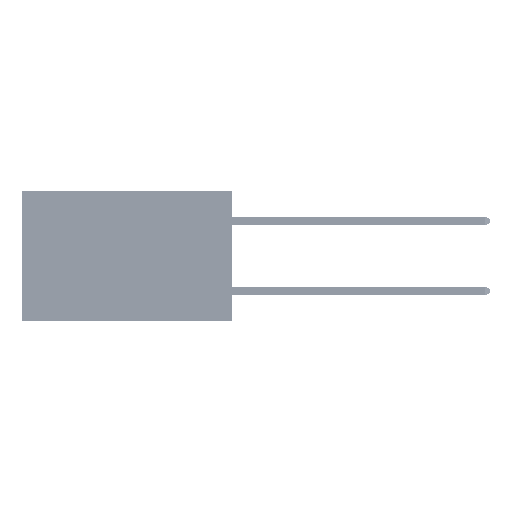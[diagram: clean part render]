
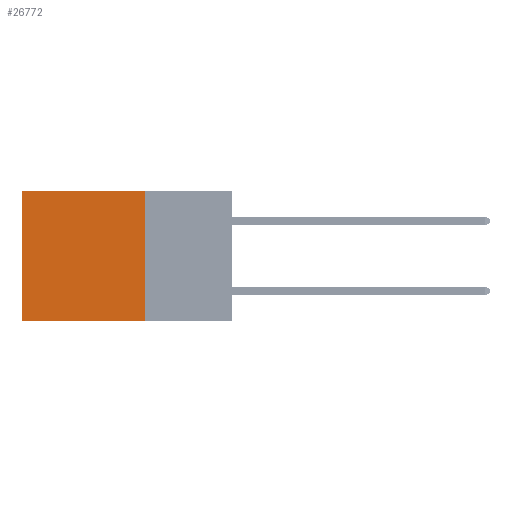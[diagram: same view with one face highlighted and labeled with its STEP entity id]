
A CAD part, left-side view. The second image highlights one B-rep face of the part: STEP entity #26772.
In plain terms, the highlighted planar face has unit normal (-1, 0, 0).
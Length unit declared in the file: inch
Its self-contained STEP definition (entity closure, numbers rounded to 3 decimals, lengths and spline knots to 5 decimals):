
#1401 = LINE ( 'NONE', #15928, #24816 ) ;
#1946 = AXIS2_PLACEMENT_3D ( 'NONE', #35711, #35251, #28089 ) ;
#4769 = ORIENTED_EDGE ( 'NONE', *, *, #20367, .F. ) ;
#4909 = CARTESIAN_POINT ( 'NONE',  ( 0.2875, 0.25, -0.37 ) ) ;
#7418 = EDGE_CURVE ( 'NONE', #21669, #17440, #38438, .T. ) ;
#8050 = EDGE_LOOP ( 'NONE', ( #38858, #29986, #4769, #27106 ) ) ;
#8296 = VERTEX_POINT ( 'NONE', #4909 ) ;
#8404 = DIRECTION ( 'NONE',  ( 0., 1., 0. ) ) ;
#8868 = CARTESIAN_POINT ( 'NONE',  ( 0.2875, 0.25, 0. ) ) ;
#14038 = VERTEX_POINT ( 'NONE', #43383 ) ;
#14043 = CARTESIAN_POINT ( 'NONE',  ( 0.2875, 0.6, 0. ) ) ;
#15928 = CARTESIAN_POINT ( 'NONE',  ( 0.2875, 0.25, -0.37 ) ) ;
#17440 = VERTEX_POINT ( 'NONE', #37973 ) ;
#18026 = EDGE_CURVE ( 'NONE', #17440, #14038, #46707, .T. ) ;
#18798 = VECTOR ( 'NONE', #8404, 39.37008 ) ;
#20367 = EDGE_CURVE ( 'NONE', #21669, #8296, #30829, .T. ) ;
#21669 = VERTEX_POINT ( 'NONE', #40233 ) ;
#23200 = CARTESIAN_POINT ( 'NONE',  ( 0.2875, 0.25, 0. ) ) ;
#24816 = VECTOR ( 'NONE', #45004, 39.37008 ) ;
#26772 = ADVANCED_FACE ( 'NONE', ( #31207 ), #46192, .F. ) ;
#27106 = ORIENTED_EDGE ( 'NONE', *, *, #7418, .T. ) ;
#28089 = DIRECTION ( 'NONE',  ( 0., 0., -1. ) ) ;
#28594 = DIRECTION ( 'NONE',  ( 0., 0., -1. ) ) ;
#29986 = ORIENTED_EDGE ( 'NONE', *, *, #46075, .F. ) ;
#30829 = LINE ( 'NONE', #23200, #34383 ) ;
#31207 = FACE_OUTER_BOUND ( 'NONE', #8050, .T. ) ;
#32213 = VECTOR ( 'NONE', #28594, 39.37008 ) ;
#34383 = VECTOR ( 'NONE', #44430, 39.37008 ) ;
#35251 = DIRECTION ( 'NONE',  ( 1., 0., 0. ) ) ;
#35711 = CARTESIAN_POINT ( 'NONE',  ( 0.2875, 0.25, 0. ) ) ;
#37973 = CARTESIAN_POINT ( 'NONE',  ( 0.2875, 0.6, 0. ) ) ;
#38438 = LINE ( 'NONE', #8868, #18798 ) ;
#38858 = ORIENTED_EDGE ( 'NONE', *, *, #18026, .T. ) ;
#40233 = CARTESIAN_POINT ( 'NONE',  ( 0.2875, 0.25, 0. ) ) ;
#43383 = CARTESIAN_POINT ( 'NONE',  ( 0.2875, 0.6, -0.37 ) ) ;
#44430 = DIRECTION ( 'NONE',  ( 0., 0., -1. ) ) ;
#45004 = DIRECTION ( 'NONE',  ( 0., 1., 0. ) ) ;
#46075 = EDGE_CURVE ( 'NONE', #8296, #14038, #1401, .T. ) ;
#46192 = PLANE ( 'NONE',  #1946 ) ;
#46707 = LINE ( 'NONE', #14043, #32213 ) ;
